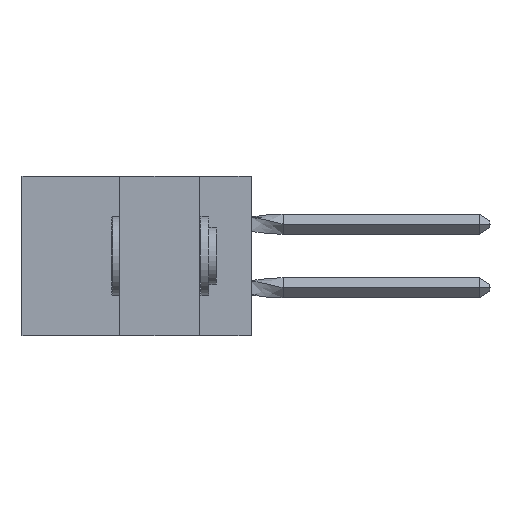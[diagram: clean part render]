
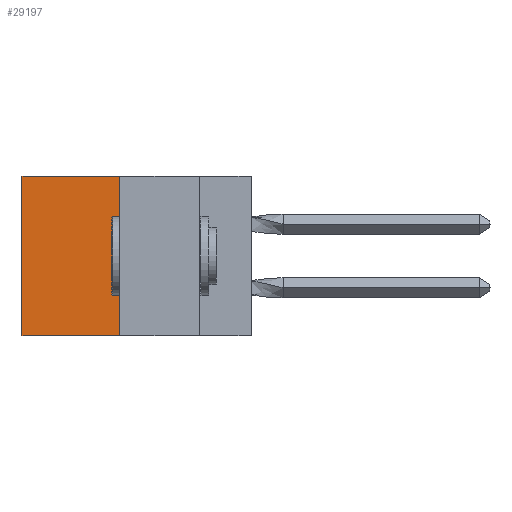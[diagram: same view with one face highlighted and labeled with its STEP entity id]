
A CAD part, left-side view. The second image highlights one B-rep face of the part: STEP entity #29197.
In plain terms, the highlighted planar face has unit normal (-1, 0, 0).
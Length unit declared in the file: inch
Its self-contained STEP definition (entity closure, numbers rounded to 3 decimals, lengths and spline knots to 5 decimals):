
#272 = ORIENTED_EDGE ( 'NONE', *, *, #12622, .T. ) ;
#502 = LINE ( 'NONE', #13464, #12978 ) ;
#1263 = DIRECTION ( 'NONE',  ( 0., 0., -1. ) ) ;
#1514 = EDGE_CURVE ( 'NONE', #4693, #28305, #17555, .T. ) ;
#2642 = CARTESIAN_POINT ( 'NONE',  ( 0.305, 0.413, 0. ) ) ;
#4693 = VERTEX_POINT ( 'NONE', #29039 ) ;
#6971 = ORIENTED_EDGE ( 'NONE', *, *, #1514, .T. ) ;
#7259 = DIRECTION ( 'NONE',  ( 0., 1., 0. ) ) ;
#7889 = VERTEX_POINT ( 'NONE', #12889 ) ;
#9347 = LINE ( 'NONE', #29472, #21035 ) ;
#9752 = ORIENTED_EDGE ( 'NONE', *, *, #28105, .F. ) ;
#12622 = EDGE_CURVE ( 'NONE', #28305, #7889, #29683, .T. ) ;
#12889 = CARTESIAN_POINT ( 'NONE',  ( 0.305, 0.72, -0.5 ) ) ;
#12978 = VECTOR ( 'NONE', #25787, 39.37008 ) ;
#13041 = VERTEX_POINT ( 'NONE', #27221 ) ;
#13464 = CARTESIAN_POINT ( 'NONE',  ( 0.305, 0.413, -0.5 ) ) ;
#14374 = CARTESIAN_POINT ( 'NONE',  ( 0.305, 0.72, 0. ) ) ;
#14664 = VECTOR ( 'NONE', #7259, 39.37008 ) ;
#15495 = DIRECTION ( 'NONE',  ( 0., 0., -1. ) ) ;
#17555 = LINE ( 'NONE', #2642, #14664 ) ;
#18509 = EDGE_LOOP ( 'NONE', ( #272, #29275, #9752, #6971 ) ) ;
#18929 = EDGE_CURVE ( 'NONE', #13041, #7889, #502, .T. ) ;
#20873 = DIRECTION ( 'NONE',  ( 0., 0., -1. ) ) ;
#21035 = VECTOR ( 'NONE', #1263, 39.37008 ) ;
#21076 = CARTESIAN_POINT ( 'NONE',  ( 0.305, 0.72, -0.5 ) ) ;
#22751 = AXIS2_PLACEMENT_3D ( 'NONE', #24730, #29469, #15495 ) ;
#23441 = VECTOR ( 'NONE', #20873, 39.37008 ) ;
#24730 = CARTESIAN_POINT ( 'NONE',  ( 0.305, 0.413, -0.5 ) ) ;
#25705 = FACE_OUTER_BOUND ( 'NONE', #18509, .T. ) ;
#25787 = DIRECTION ( 'NONE',  ( 0., 1., 0. ) ) ;
#27221 = CARTESIAN_POINT ( 'NONE',  ( 0.305, 0.413, -0.5 ) ) ;
#28105 = EDGE_CURVE ( 'NONE', #4693, #13041, #9347, .T. ) ;
#28305 = VERTEX_POINT ( 'NONE', #14374 ) ;
#29039 = CARTESIAN_POINT ( 'NONE',  ( 0.305, 0.413, 0. ) ) ;
#29197 = ADVANCED_FACE ( 'NONE', ( #25705 ), #29574, .F. ) ;
#29275 = ORIENTED_EDGE ( 'NONE', *, *, #18929, .F. ) ;
#29469 = DIRECTION ( 'NONE',  ( 1., 0., 0. ) ) ;
#29472 = CARTESIAN_POINT ( 'NONE',  ( 0.305, 0.413, -0.5 ) ) ;
#29574 = PLANE ( 'NONE',  #22751 ) ;
#29683 = LINE ( 'NONE', #21076, #23441 ) ;
